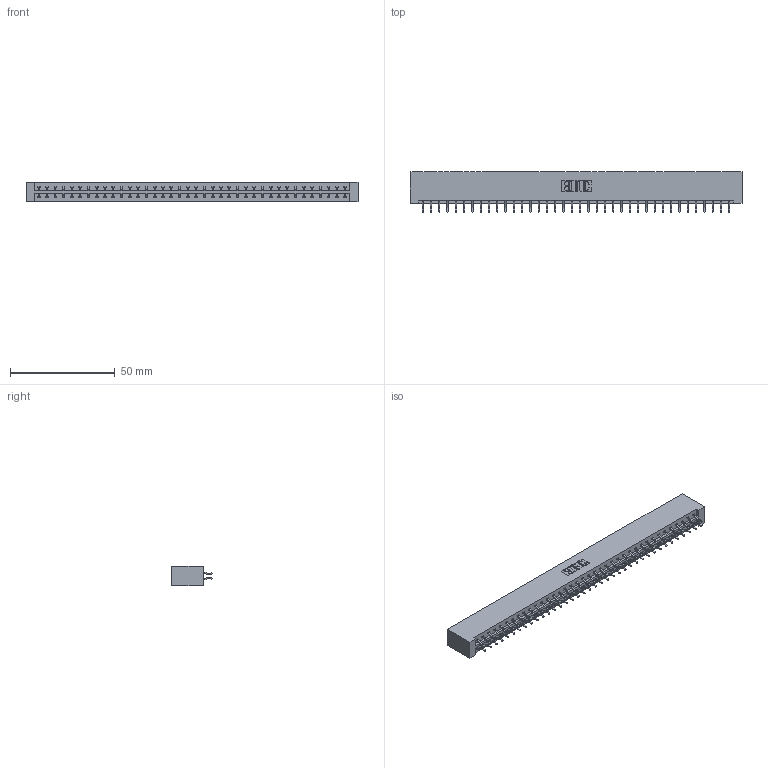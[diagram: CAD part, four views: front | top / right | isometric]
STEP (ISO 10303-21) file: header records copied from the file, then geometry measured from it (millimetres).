
FILE_DESCRIPTION (( 'STEP AP203' ), '1' );
FILE_NAME ('333-076-556-201.STEP', '2018-08-04T23:23:50', ( '' ), ( '' ), 'SwSTEP 2.0', 'SolidWorks 2016', '' );
FILE_SCHEMA (( 'CONFIG_CONTROL_DESIGN' ));
Length unit declared in the file: inch
Products named in the file (3): 333 Part_Lugless; 345-292-001_556 Tail; 333-076-556-201
Assembly tree (77 placements, depth 2):
  333-076-556-201
    333 Part_Lugless
    345-292-001_556 Tail  x76
Bounding box: 158.83 x 19.57 x 9.4 mm (x, y, z)
Volume: 16807.1 mm3; surface area: 19776.5 mm2
Topology: 77 solids, 77 shells, 4514 faces, 13435 edges, 8854 vertices
Faces by surface type: plane 3106, cylinder 1408
Entity records: 24907 total; most frequent: CARTESIAN_POINT 4146, ORIENTED_EDGE 4070, DIRECTION 3531, EDGE_CURVE 2035, LINE 1907, VECTOR 1907, VERTEX_POINT 1354, AXIS2_PLACEMENT_3D 812
